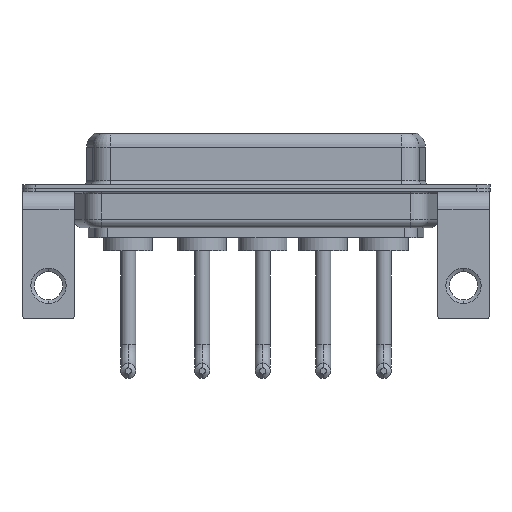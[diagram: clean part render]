
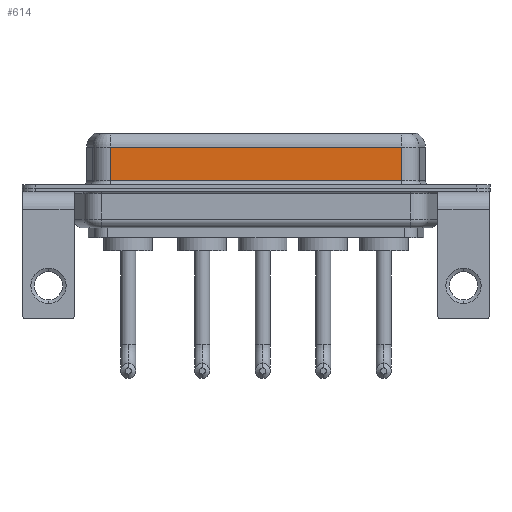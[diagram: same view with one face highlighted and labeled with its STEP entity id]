
A CAD part, front view. The second image highlights one B-rep face of the part: STEP entity #614.
In plain terms, the highlighted planar face has unit normal (0, -1, 0).
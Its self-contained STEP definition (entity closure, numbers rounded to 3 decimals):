
#548 = VERTEX_POINT ( 'NONE', #5854 ) ;
#614 = ADVANCED_FACE ( 'NONE', ( #6181 ), #10484, .F. ) ;
#814 = ORIENTED_EDGE ( 'NONE', *, *, #11636, .F. ) ;
#1152 = CARTESIAN_POINT ( 'NONE',  ( 40.037, -3.95, 6.4 ) ) ;
#1278 = VECTOR ( 'NONE', #7302, 1000. ) ;
#1531 = VERTEX_POINT ( 'NONE', #10240 ) ;
#1686 = LINE ( 'NONE', #10887, #9975 ) ;
#1779 = DIRECTION ( 'NONE',  ( -1., 0., 0. ) ) ;
#1958 = EDGE_CURVE ( 'NONE', #548, #1531, #12157, .T. ) ;
#2489 = AXIS2_PLACEMENT_3D ( 'NONE', #1152, #9105, #3123 ) ;
#3123 = DIRECTION ( 'NONE',  ( 0., 0., 1. ) ) ;
#3195 = EDGE_CURVE ( 'NONE', #1531, #7008, #1686, .T. ) ;
#5135 = CARTESIAN_POINT ( 'NONE',  ( 40.037, -3.95, 6.4 ) ) ;
#5136 = ORIENTED_EDGE ( 'NONE', *, *, #5426, .T. ) ;
#5389 = ORIENTED_EDGE ( 'NONE', *, *, #3195, .T. ) ;
#5426 = EDGE_CURVE ( 'NONE', #7008, #10389, #13292, .T. ) ;
#5724 = CARTESIAN_POINT ( 'NONE',  ( 40.037, -3.95, 0.9 ) ) ;
#5834 = DIRECTION ( 'NONE',  ( 0., 0., -1. ) ) ;
#5854 = CARTESIAN_POINT ( 'NONE',  ( 40.037, -3.95, 4.65 ) ) ;
#6106 = DIRECTION ( 'NONE',  ( 1., 0., 0. ) ) ;
#6181 = FACE_OUTER_BOUND ( 'NONE', #10493, .T. ) ;
#7008 = VERTEX_POINT ( 'NONE', #9314 ) ;
#7038 = VECTOR ( 'NONE', #6106, 1000. ) ;
#7302 = DIRECTION ( 'NONE',  ( 0., 0., -1. ) ) ;
#7552 = ORIENTED_EDGE ( 'NONE', *, *, #1958, .T. ) ;
#9105 = DIRECTION ( 'NONE',  ( 0., 1., 0. ) ) ;
#9314 = CARTESIAN_POINT ( 'NONE',  ( 7.013, -3.95, 0.9 ) ) ;
#9975 = VECTOR ( 'NONE', #5834, 1000. ) ;
#10207 = CARTESIAN_POINT ( 'NONE',  ( 40.037, -3.95, 0.9 ) ) ;
#10240 = CARTESIAN_POINT ( 'NONE',  ( 7.013, -3.95, 4.65 ) ) ;
#10389 = VERTEX_POINT ( 'NONE', #5724 ) ;
#10484 = PLANE ( 'NONE',  #2489 ) ;
#10493 = EDGE_LOOP ( 'NONE', ( #814, #7552, #5389, #5136 ) ) ;
#10887 = CARTESIAN_POINT ( 'NONE',  ( 7.013, -3.95, 6.4 ) ) ;
#11636 = EDGE_CURVE ( 'NONE', #548, #10389, #13333, .T. ) ;
#12157 = LINE ( 'NONE', #12220, #13082 ) ;
#12220 = CARTESIAN_POINT ( 'NONE',  ( 40.037, -3.95, 4.65 ) ) ;
#13082 = VECTOR ( 'NONE', #1779, 1000. ) ;
#13292 = LINE ( 'NONE', #10207, #7038 ) ;
#13333 = LINE ( 'NONE', #5135, #1278 ) ;
